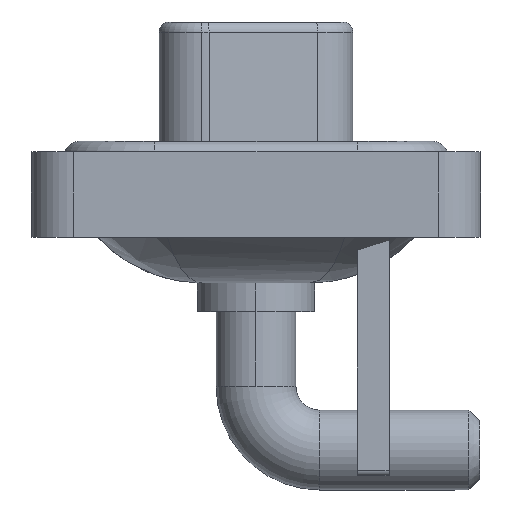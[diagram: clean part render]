
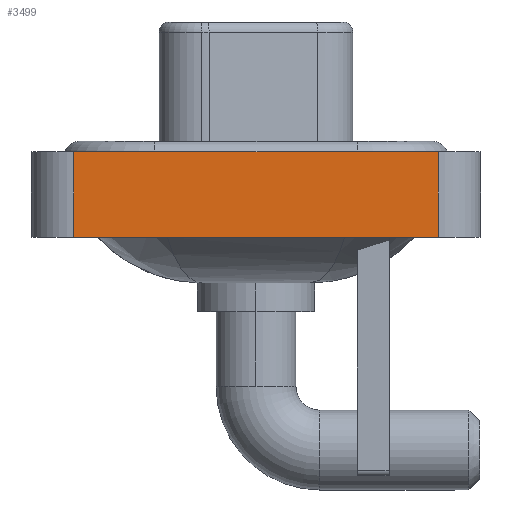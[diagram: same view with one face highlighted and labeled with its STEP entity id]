
A CAD part, left-side view. The second image highlights one B-rep face of the part: STEP entity #3499.
In plain terms, the highlighted planar face has unit normal (-1, 0, 0).
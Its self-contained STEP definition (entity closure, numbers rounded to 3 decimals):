
#373 = DIRECTION ( 'NONE',  ( 0., -1., 0. ) ) ;
#550 = CARTESIAN_POINT ( 'NONE',  ( -7.25, 8.55, -3.6 ) ) ;
#600 = EDGE_CURVE ( 'NONE', #2661, #7455, #6021, .T. ) ;
#1059 = AXIS2_PLACEMENT_3D ( 'NONE', #13159, #15793, #11645 ) ;
#1318 = DIRECTION ( 'NONE',  ( 0., -1., 0. ) ) ;
#2026 = DIRECTION ( 'NONE',  ( 0., 0., 1. ) ) ;
#2661 = VERTEX_POINT ( 'NONE', #15039 ) ;
#2728 = VERTEX_POINT ( 'NONE', #3521 ) ;
#2731 = EDGE_LOOP ( 'NONE', ( #12784, #3351, #7206, #13766 ) ) ;
#3351 = ORIENTED_EDGE ( 'NONE', *, *, #11746, .F. ) ;
#3469 = CARTESIAN_POINT ( 'NONE',  ( -7.25, -8.55, -3.6 ) ) ;
#3499 = ADVANCED_FACE ( 'NONE', ( #11554 ), #17569, .T. ) ;
#3521 = CARTESIAN_POINT ( 'NONE',  ( -7.25, -8.55, 0.4 ) ) ;
#4330 = VERTEX_POINT ( 'NONE', #12688 ) ;
#4984 = LINE ( 'NONE', #3469, #12787 ) ;
#6021 = LINE ( 'NONE', #550, #17377 ) ;
#6821 = EDGE_CURVE ( 'NONE', #2661, #4330, #4984, .T. ) ;
#7206 = ORIENTED_EDGE ( 'NONE', *, *, #600, .F. ) ;
#7455 = VERTEX_POINT ( 'NONE', #9407 ) ;
#8506 = LINE ( 'NONE', #18404, #16661 ) ;
#9407 = CARTESIAN_POINT ( 'NONE',  ( -7.25, 8.55, 0.4 ) ) ;
#10257 = CARTESIAN_POINT ( 'NONE',  ( -7.25, -8.55, -3.6 ) ) ;
#11554 = FACE_OUTER_BOUND ( 'NONE', #2731, .T. ) ;
#11645 = DIRECTION ( 'NONE',  ( 0., 0., 1. ) ) ;
#11746 = EDGE_CURVE ( 'NONE', #7455, #2728, #8506, .T. ) ;
#12688 = CARTESIAN_POINT ( 'NONE',  ( -7.25, -8.55, -3.6 ) ) ;
#12784 = ORIENTED_EDGE ( 'NONE', *, *, #17403, .T. ) ;
#12787 = VECTOR ( 'NONE', #373, 1000. ) ;
#13159 = CARTESIAN_POINT ( 'NONE',  ( -7.25, -8.55, -3.6 ) ) ;
#13766 = ORIENTED_EDGE ( 'NONE', *, *, #6821, .T. ) ;
#14804 = VECTOR ( 'NONE', #2026, 1000. ) ;
#14958 = LINE ( 'NONE', #10257, #14804 ) ;
#14992 = DIRECTION ( 'NONE',  ( 0., 0., 1. ) ) ;
#15039 = CARTESIAN_POINT ( 'NONE',  ( -7.25, 8.55, -3.6 ) ) ;
#15793 = DIRECTION ( 'NONE',  ( -1., 0., 0. ) ) ;
#16661 = VECTOR ( 'NONE', #1318, 1000. ) ;
#17377 = VECTOR ( 'NONE', #14992, 1000. ) ;
#17403 = EDGE_CURVE ( 'NONE', #4330, #2728, #14958, .T. ) ;
#17569 = PLANE ( 'NONE',  #1059 ) ;
#18404 = CARTESIAN_POINT ( 'NONE',  ( -7.25, -8.55, 0.4 ) ) ;
